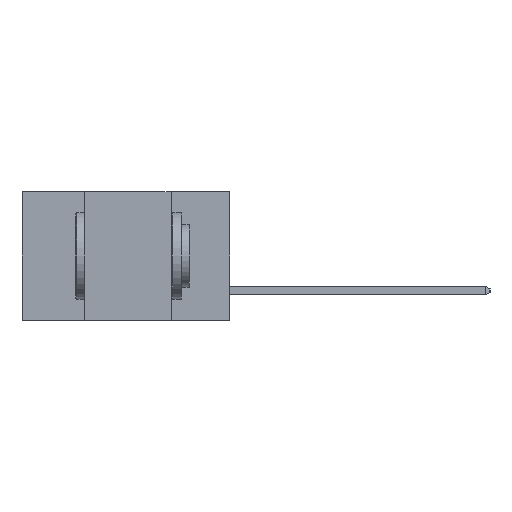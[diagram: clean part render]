
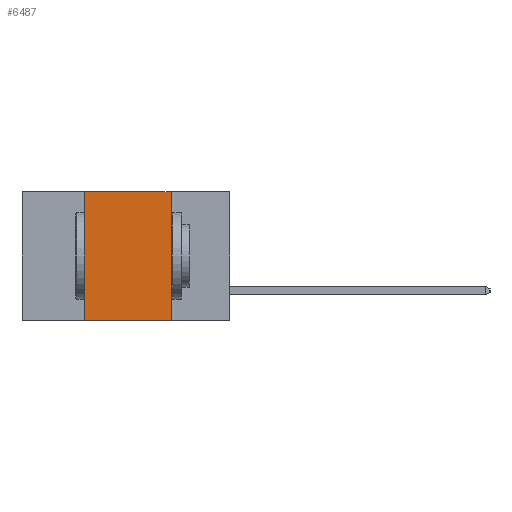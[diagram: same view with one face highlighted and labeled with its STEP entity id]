
A CAD part, left-side view. The second image highlights one B-rep face of the part: STEP entity #6487.
In plain terms, the highlighted planar face has unit normal (-1, 0, 0).
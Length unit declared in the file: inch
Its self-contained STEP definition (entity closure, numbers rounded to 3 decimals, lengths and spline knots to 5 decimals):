
#977 = ORIENTED_EDGE ( 'NONE', *, *, #1849, .F. ) ;
#1010 = CARTESIAN_POINT ( 'NONE',  ( 0., 0.17, -0.37 ) ) ;
#1167 = CARTESIAN_POINT ( 'NONE',  ( 0., 0.42, -0.37 ) ) ;
#1849 = EDGE_CURVE ( 'NONE', #9230, #3703, #12012, .T. ) ;
#1956 = VECTOR ( 'NONE', #12517, 39.37008 ) ;
#2432 = ORIENTED_EDGE ( 'NONE', *, *, #12701, .T. ) ;
#3121 = VERTEX_POINT ( 'NONE', #4345 ) ;
#3251 = EDGE_CURVE ( 'NONE', #3703, #3121, #11344, .T. ) ;
#3338 = CARTESIAN_POINT ( 'NONE',  ( 0., 0.42, 0. ) ) ;
#3355 = DIRECTION ( 'NONE',  ( 0., 0., 1. ) ) ;
#3681 = LINE ( 'NONE', #7101, #6363 ) ;
#3703 = VERTEX_POINT ( 'NONE', #3338 ) ;
#4024 = PLANE ( 'NONE',  #11714 ) ;
#4345 = CARTESIAN_POINT ( 'NONE',  ( 0., 0.17, 0. ) ) ;
#4650 = ORIENTED_EDGE ( 'NONE', *, *, #3251, .F. ) ;
#5023 = DIRECTION ( 'NONE',  ( 1., 0., 0. ) ) ;
#5297 = EDGE_CURVE ( 'NONE', #3121, #8185, #3681, .T. ) ;
#6354 = ORIENTED_EDGE ( 'NONE', *, *, #5297, .F. ) ;
#6363 = VECTOR ( 'NONE', #12783, 39.37008 ) ;
#6487 = ADVANCED_FACE ( 'NONE', ( #7600 ), #4024, .F. ) ;
#7101 = CARTESIAN_POINT ( 'NONE',  ( 0., 0.17, -0.37 ) ) ;
#7600 = FACE_OUTER_BOUND ( 'NONE', #10891, .T. ) ;
#8185 = VERTEX_POINT ( 'NONE', #1010 ) ;
#8562 = DIRECTION ( 'NONE',  ( 0., -1., 0. ) ) ;
#8803 = CARTESIAN_POINT ( 'NONE',  ( 0., 0.6, 0. ) ) ;
#8964 = CARTESIAN_POINT ( 'NONE',  ( 0., 0.6, 0. ) ) ;
#9230 = VERTEX_POINT ( 'NONE', #1167 ) ;
#9950 = LINE ( 'NONE', #10636, #1956 ) ;
#10636 = CARTESIAN_POINT ( 'NONE',  ( 0., 0.6, -0.37 ) ) ;
#10711 = VECTOR ( 'NONE', #8562, 39.37008 ) ;
#10891 = EDGE_LOOP ( 'NONE', ( #6354, #4650, #977, #2432 ) ) ;
#11338 = CARTESIAN_POINT ( 'NONE',  ( 0., 0.42, -0.37 ) ) ;
#11344 = LINE ( 'NONE', #8803, #10711 ) ;
#11439 = VECTOR ( 'NONE', #3355, 39.37008 ) ;
#11714 = AXIS2_PLACEMENT_3D ( 'NONE', #8964, #5023, #11938 ) ;
#11938 = DIRECTION ( 'NONE',  ( 0., 0., -1. ) ) ;
#12012 = LINE ( 'NONE', #11338, #11439 ) ;
#12517 = DIRECTION ( 'NONE',  ( 0., -1., 0. ) ) ;
#12701 = EDGE_CURVE ( 'NONE', #9230, #8185, #9950, .T. ) ;
#12783 = DIRECTION ( 'NONE',  ( 0., 0., -1. ) ) ;
